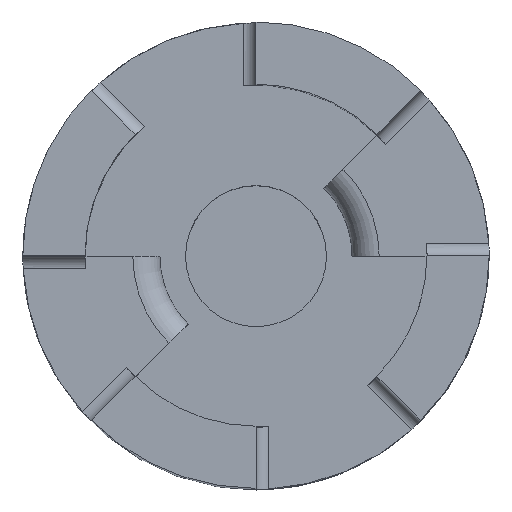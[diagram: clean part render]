
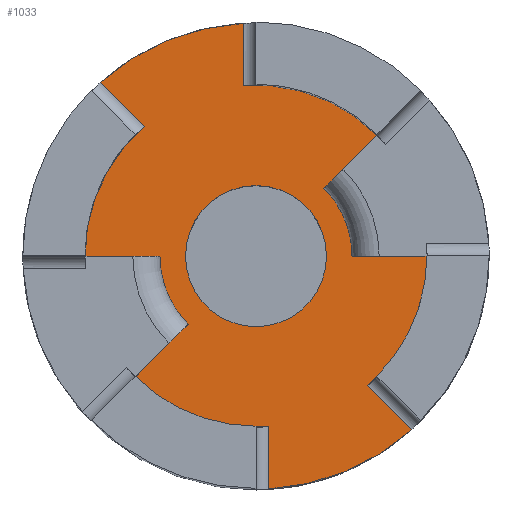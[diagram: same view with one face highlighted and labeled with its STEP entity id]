
A CAD part, top view. The second image highlights one B-rep face of the part: STEP entity #1033.
In plain terms, the highlighted planar face has unit normal (0, 0, 1).
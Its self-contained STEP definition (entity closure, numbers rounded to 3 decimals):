
#17=FACE_BOUND('',#160,.T.);
#53=PLANE('',#1154);
#102=FACE_OUTER_BOUND('',#159,.T.);
#159=EDGE_LOOP('',(#864,#865,#866,#867,#868,#869,#870,#871,#872,#873,#874,
#875,#876,#877,#878,#879));
#160=EDGE_LOOP('',(#880,#881));
#183=LINE('',#1516,#267);
#190=LINE('',#1545,#274);
#239=LINE('',#1849,#323);
#242=LINE('',#1867,#326);
#244=LINE('',#1873,#328);
#245=LINE('',#1877,#329);
#246=LINE('',#1879,#330);
#247=LINE('',#1883,#331);
#267=VECTOR('',#1209,10.);
#274=VECTOR('',#1236,10.);
#323=VECTOR('',#1403,10.);
#326=VECTOR('',#1410,10.);
#328=VECTOR('',#1416,10.);
#329=VECTOR('',#1421,10.);
#330=VECTOR('',#1422,10.);
#331=VECTOR('',#1425,10.);
#348=CIRCLE('',#1074,3.302);
#349=CIRCLE('',#1075,3.302);
#366=CIRCLE('',#1105,10.922);
#374=CIRCLE('',#1113,10.922);
#394=CIRCLE('',#1155,8.01);
#395=CIRCLE('',#1156,4.5);
#396=CIRCLE('',#1157,8.01);
#397=CIRCLE('',#1158,8.01);
#398=CIRCLE('',#1159,4.5);
#399=CIRCLE('',#1160,8.01);
#404=VERTEX_POINT('',#1494);
#405=VERTEX_POINT('',#1495);
#412=VERTEX_POINT('',#1513);
#413=VERTEX_POINT('',#1515);
#424=VERTEX_POINT('',#1542);
#425=VERTEX_POINT('',#1544);
#445=VERTEX_POINT('',#1672);
#446=VERTEX_POINT('',#1683);
#461=VERTEX_POINT('',#1724);
#462=VERTEX_POINT('',#1735);
#490=VERTEX_POINT('',#1836);
#494=VERTEX_POINT('',#1856);
#495=VERTEX_POINT('',#1870);
#496=VERTEX_POINT('',#1872);
#497=VERTEX_POINT('',#1875);
#498=VERTEX_POINT('',#1878);
#499=VERTEX_POINT('',#1880);
#500=VERTEX_POINT('',#1882);
#508=EDGE_CURVE('',#404,#405,#348,.T.);
#509=EDGE_CURVE('',#405,#404,#349,.T.);
#518=EDGE_CURVE('',#413,#412,#183,.T.);
#532=EDGE_CURVE('',#425,#424,#190,.T.);
#561=EDGE_CURVE('',#446,#445,#366,.F.);
#579=EDGE_CURVE('',#462,#461,#374,.F.);
#626=EDGE_CURVE('',#462,#490,#239,.T.);
#630=EDGE_CURVE('',#494,#461,#242,.T.);
#632=EDGE_CURVE('',#494,#495,#394,.T.);
#633=EDGE_CURVE('',#495,#496,#244,.T.);
#634=EDGE_CURVE('',#425,#496,#395,.T.);
#635=EDGE_CURVE('',#424,#497,#396,.T.);
#636=EDGE_CURVE('',#446,#497,#245,.T.);
#637=EDGE_CURVE('',#498,#445,#246,.T.);
#638=EDGE_CURVE('',#498,#499,#397,.T.);
#639=EDGE_CURVE('',#499,#500,#247,.T.);
#640=EDGE_CURVE('',#413,#500,#398,.T.);
#641=EDGE_CURVE('',#412,#490,#399,.T.);
#864=ORIENTED_EDGE('',*,*,#626,.F.);
#865=ORIENTED_EDGE('',*,*,#579,.T.);
#866=ORIENTED_EDGE('',*,*,#630,.F.);
#867=ORIENTED_EDGE('',*,*,#632,.T.);
#868=ORIENTED_EDGE('',*,*,#633,.T.);
#869=ORIENTED_EDGE('',*,*,#634,.F.);
#870=ORIENTED_EDGE('',*,*,#532,.T.);
#871=ORIENTED_EDGE('',*,*,#635,.T.);
#872=ORIENTED_EDGE('',*,*,#636,.F.);
#873=ORIENTED_EDGE('',*,*,#561,.T.);
#874=ORIENTED_EDGE('',*,*,#637,.F.);
#875=ORIENTED_EDGE('',*,*,#638,.T.);
#876=ORIENTED_EDGE('',*,*,#639,.T.);
#877=ORIENTED_EDGE('',*,*,#640,.F.);
#878=ORIENTED_EDGE('',*,*,#518,.T.);
#879=ORIENTED_EDGE('',*,*,#641,.T.);
#880=ORIENTED_EDGE('',*,*,#508,.T.);
#881=ORIENTED_EDGE('',*,*,#509,.T.);
#1033=ADVANCED_FACE('',(#102,#17),#53,.T.);
#1074=AXIS2_PLACEMENT_3D('',#1496,#1188,#1189);
#1075=AXIS2_PLACEMENT_3D('',#1497,#1190,#1191);
#1105=AXIS2_PLACEMENT_3D('',#1684,#1276,#1277);
#1113=AXIS2_PLACEMENT_3D('',#1736,#1300,#1301);
#1154=AXIS2_PLACEMENT_3D('',#1869,#1412,#1413);
#1155=AXIS2_PLACEMENT_3D('',#1871,#1414,#1415);
#1156=AXIS2_PLACEMENT_3D('',#1874,#1417,#1418);
#1157=AXIS2_PLACEMENT_3D('',#1876,#1419,#1420);
#1158=AXIS2_PLACEMENT_3D('',#1881,#1423,#1424);
#1159=AXIS2_PLACEMENT_3D('',#1884,#1426,#1427);
#1160=AXIS2_PLACEMENT_3D('',#1885,#1428,#1429);
#1188=DIRECTION('center_axis',(0.,0.,-1.));
#1189=DIRECTION('ref_axis',(1.,0.,0.));
#1190=DIRECTION('center_axis',(0.,0.,-1.));
#1191=DIRECTION('ref_axis',(1.,0.,0.));
#1209=DIRECTION('',(0.707,0.707,0.));
#1236=DIRECTION('',(-0.707,-0.707,0.));
#1276=DIRECTION('center_axis',(0.,0.,-1.));
#1277=DIRECTION('ref_axis',(1.,0.,0.));
#1300=DIRECTION('center_axis',(0.,0.,-1.));
#1301=DIRECTION('ref_axis',(1.,0.,0.));
#1403=DIRECTION('',(0.,-1.,0.));
#1410=DIRECTION('',(-0.707,0.707,0.));
#1412=DIRECTION('center_axis',(0.,0.,1.));
#1413=DIRECTION('ref_axis',(1.,0.,0.));
#1414=DIRECTION('center_axis',(0.,0.,1.));
#1415=DIRECTION('ref_axis',(0.707,-0.707,0.));
#1416=DIRECTION('',(1.,0.,0.));
#1417=DIRECTION('center_axis',(0.,0.,-1.));
#1418=DIRECTION('ref_axis',(1.,0.,0.));
#1419=DIRECTION('center_axis',(0.,0.,1.));
#1420=DIRECTION('ref_axis',(0.707,-0.707,0.));
#1421=DIRECTION('',(0.,1.,0.));
#1422=DIRECTION('',(0.707,-0.707,0.));
#1423=DIRECTION('center_axis',(0.,0.,1.));
#1424=DIRECTION('ref_axis',(-0.707,0.707,0.));
#1425=DIRECTION('',(-1.,0.,0.));
#1426=DIRECTION('center_axis',(0.,0.,-1.));
#1427=DIRECTION('ref_axis',(1.,0.,0.));
#1428=DIRECTION('center_axis',(0.,0.,1.));
#1429=DIRECTION('ref_axis',(-0.707,0.707,0.));
#1494=CARTESIAN_POINT('',(3.302,0.,2.54));
#1495=CARTESIAN_POINT('',(-3.302,0.,2.54));
#1496=CARTESIAN_POINT('Origin',(0.,0.,2.54));
#1497=CARTESIAN_POINT('Origin',(0.,0.,2.54));
#1513=CARTESIAN_POINT('',(5.664,5.664,2.54));
#1515=CARTESIAN_POINT('',(3.182,3.182,2.54));
#1516=CARTESIAN_POINT('',(2.832,2.832,2.54));
#1542=CARTESIAN_POINT('',(-5.664,-5.664,2.54));
#1544=CARTESIAN_POINT('',(-3.182,-3.182,2.54));
#1545=CARTESIAN_POINT('',(-2.832,-2.832,2.54));
#1672=CARTESIAN_POINT('',(7.287,-8.136,2.54));
#1683=CARTESIAN_POINT('',(0.6,-10.906,2.54));
#1684=CARTESIAN_POINT('Origin',(0.,0.,2.54));
#1724=CARTESIAN_POINT('',(-7.287,8.136,2.54));
#1735=CARTESIAN_POINT('',(-0.6,10.906,2.54));
#1736=CARTESIAN_POINT('Origin',(0.,0.,2.54));
#1836=CARTESIAN_POINT('',(-0.6,7.987,2.54));
#1849=CARTESIAN_POINT('',(-0.6,5.08,2.54));
#1856=CARTESIAN_POINT('',(-5.224,6.072,2.54));
#1867=CARTESIAN_POINT('',(-2.408,3.256,2.54));
#1869=CARTESIAN_POINT('Origin',(0.,0.,
2.54));
#1870=CARTESIAN_POINT('',(-8.01,0.,2.54));
#1871=CARTESIAN_POINT('Origin',(0.,0.,
2.54));
#1872=CARTESIAN_POINT('',(-4.5,0.,2.54));
#1873=CARTESIAN_POINT('',(-1.594,0.,2.54));
#1874=CARTESIAN_POINT('Origin',(0.,0.,2.54));
#1875=CARTESIAN_POINT('',(0.6,-7.987,2.54));
#1876=CARTESIAN_POINT('Origin',(0.,0.,
2.54));
#1877=CARTESIAN_POINT('',(0.6,-5.08,2.54));
#1878=CARTESIAN_POINT('',(5.224,-6.072,2.54));
#1879=CARTESIAN_POINT('',(2.408,-3.256,2.54));
#1880=CARTESIAN_POINT('',(8.01,0.,2.54));
#1881=CARTESIAN_POINT('Origin',(0.,0.,
2.54));
#1882=CARTESIAN_POINT('',(4.5,0.,2.54));
#1883=CARTESIAN_POINT('',(1.594,0.,2.54));
#1884=CARTESIAN_POINT('Origin',(0.,0.,2.54));
#1885=CARTESIAN_POINT('Origin',(0.,0.,
2.54));
